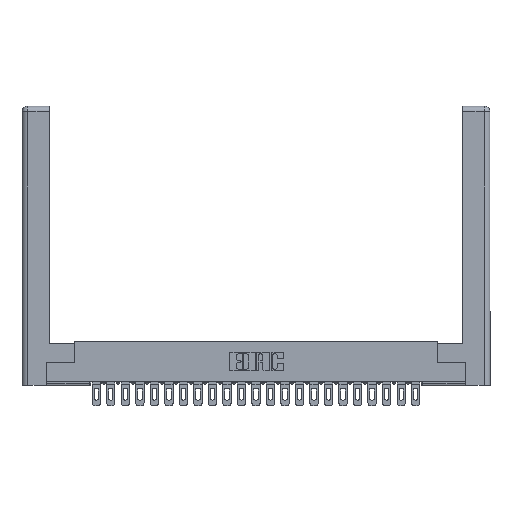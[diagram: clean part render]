
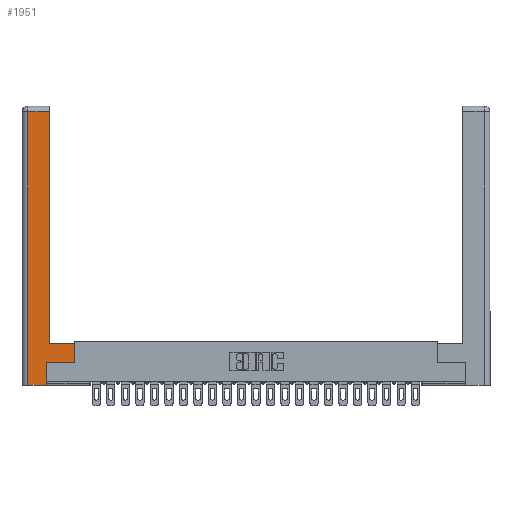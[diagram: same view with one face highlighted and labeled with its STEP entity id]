
A CAD part, top view. The second image highlights one B-rep face of the part: STEP entity #1951.
In plain terms, the highlighted planar face has unit normal (0, 0, 1).
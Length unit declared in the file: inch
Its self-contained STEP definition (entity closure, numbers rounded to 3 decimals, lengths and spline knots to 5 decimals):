
#89 = EDGE_CURVE ( 'NONE', #23051, #14105, #11662, .T. ) ;
#340 = ORIENTED_EDGE ( 'NONE', *, *, #14212, .T. ) ;
#574 = CARTESIAN_POINT ( 'NONE',  ( 0.0615, 0., 0. ) ) ;
#1230 = EDGE_CURVE ( 'NONE', #1372, #14153, #24521, .T. ) ;
#1372 = VERTEX_POINT ( 'NONE', #574 ) ;
#1722 = EDGE_LOOP ( 'NONE', ( #20308, #12429, #10786, #2805, #340, #14926, #14289, #20986 ) ) ;
#1798 = CARTESIAN_POINT ( 'NONE',  ( 0.295, 0.45, 0. ) ) ;
#1951 = ADVANCED_FACE ( 'NONE', ( #19927 ), #13357, .F. ) ;
#1955 = DIRECTION ( 'NONE',  ( 1., 0., 0. ) ) ;
#2156 = CARTESIAN_POINT ( 'NONE',  ( 0.295, 2.94, 0. ) ) ;
#2805 = ORIENTED_EDGE ( 'NONE', *, *, #1230, .T. ) ;
#2895 = VECTOR ( 'NONE', #10157, 39.37008 ) ;
#4245 = DIRECTION ( 'NONE',  ( 1., 0., 0. ) ) ;
#4495 = CARTESIAN_POINT ( 'NONE',  ( 0.265, 0., 0. ) ) ;
#4953 = VERTEX_POINT ( 'NONE', #10682 ) ;
#5195 = VECTOR ( 'NONE', #1955, 39.37008 ) ;
#5208 = CARTESIAN_POINT ( 'NONE',  ( 0.0615, 2.94, 0. ) ) ;
#5622 = CARTESIAN_POINT ( 'NONE',  ( 0.0615, 2.94, 0. ) ) ;
#5957 = DIRECTION ( 'NONE',  ( 0., 1., 0. ) ) ;
#7594 = VECTOR ( 'NONE', #4245, 39.37008 ) ;
#7850 = LINE ( 'NONE', #10417, #20160 ) ;
#8403 = AXIS2_PLACEMENT_3D ( 'NONE', #17326, #23105, #17247 ) ;
#8462 = LINE ( 'NONE', #5622, #2895 ) ;
#8598 = DIRECTION ( 'NONE',  ( 0., 1., 0. ) ) ;
#8698 = CARTESIAN_POINT ( 'NONE',  ( 0.565, 0.45, 0. ) ) ;
#9253 = EDGE_CURVE ( 'NONE', #23744, #18658, #18318, .T. ) ;
#9287 = EDGE_CURVE ( 'NONE', #18658, #18947, #8462, .T. ) ;
#10000 = CARTESIAN_POINT ( 'NONE',  ( 0.565, 0.245, 0. ) ) ;
#10157 = DIRECTION ( 'NONE',  ( -1., 0., 0. ) ) ;
#10417 = CARTESIAN_POINT ( 'NONE',  ( 0.265, 0.245, 0. ) ) ;
#10682 = CARTESIAN_POINT ( 'NONE',  ( 0.565, 0.45, 0. ) ) ;
#10683 = DIRECTION ( 'NONE',  ( 0., 1., 0. ) ) ;
#10786 = ORIENTED_EDGE ( 'NONE', *, *, #11906, .T. ) ;
#11428 = DIRECTION ( 'NONE',  ( -1., 0., 0. ) ) ;
#11662 = LINE ( 'NONE', #19858, #5195 ) ;
#11906 = EDGE_CURVE ( 'NONE', #18947, #1372, #14432, .T. ) ;
#12325 = VECTOR ( 'NONE', #11428, 39.37008 ) ;
#12429 = ORIENTED_EDGE ( 'NONE', *, *, #9287, .T. ) ;
#13256 = LINE ( 'NONE', #1798, #12325 ) ;
#13357 = PLANE ( 'NONE',  #8403 ) ;
#13699 = VECTOR ( 'NONE', #5957, 39.37008 ) ;
#14105 = VERTEX_POINT ( 'NONE', #10000 ) ;
#14153 = VERTEX_POINT ( 'NONE', #4495 ) ;
#14212 = EDGE_CURVE ( 'NONE', #14153, #23051, #7850, .T. ) ;
#14289 = ORIENTED_EDGE ( 'NONE', *, *, #22937, .T. ) ;
#14432 = LINE ( 'NONE', #21967, #17833 ) ;
#14926 = ORIENTED_EDGE ( 'NONE', *, *, #89, .T. ) ;
#15078 = CARTESIAN_POINT ( 'NONE',  ( 0.265, 0.245, 0. ) ) ;
#17247 = DIRECTION ( 'NONE',  ( -1., 0., 0. ) ) ;
#17326 = CARTESIAN_POINT ( 'NONE',  ( 0., 0., 0. ) ) ;
#17833 = VECTOR ( 'NONE', #19698, 39.37008 ) ;
#18143 = LINE ( 'NONE', #8698, #22169 ) ;
#18318 = LINE ( 'NONE', #21747, #13699 ) ;
#18658 = VERTEX_POINT ( 'NONE', #2156 ) ;
#18947 = VERTEX_POINT ( 'NONE', #5208 ) ;
#19077 = CARTESIAN_POINT ( 'NONE',  ( 0.295, 0.45, 0. ) ) ;
#19698 = DIRECTION ( 'NONE',  ( 0., -1., 0. ) ) ;
#19858 = CARTESIAN_POINT ( 'NONE',  ( 0.565, 0.245, 0. ) ) ;
#19927 = FACE_OUTER_BOUND ( 'NONE', #1722, .T. ) ;
#20160 = VECTOR ( 'NONE', #8598, 39.37008 ) ;
#20308 = ORIENTED_EDGE ( 'NONE', *, *, #9253, .T. ) ;
#20986 = ORIENTED_EDGE ( 'NONE', *, *, #21929, .T. ) ;
#21747 = CARTESIAN_POINT ( 'NONE',  ( 0.295, 3., 0. ) ) ;
#21929 = EDGE_CURVE ( 'NONE', #4953, #23744, #13256, .T. ) ;
#21967 = CARTESIAN_POINT ( 'NONE',  ( 0.0615, 0., 0. ) ) ;
#22169 = VECTOR ( 'NONE', #10683, 39.37008 ) ;
#22937 = EDGE_CURVE ( 'NONE', #14105, #4953, #18143, .T. ) ;
#23051 = VERTEX_POINT ( 'NONE', #15078 ) ;
#23105 = DIRECTION ( 'NONE',  ( 0., 0., -1. ) ) ;
#23744 = VERTEX_POINT ( 'NONE', #19077 ) ;
#23774 = CARTESIAN_POINT ( 'NONE',  ( 0.265, 0., 0. ) ) ;
#24521 = LINE ( 'NONE', #23774, #7594 ) ;
